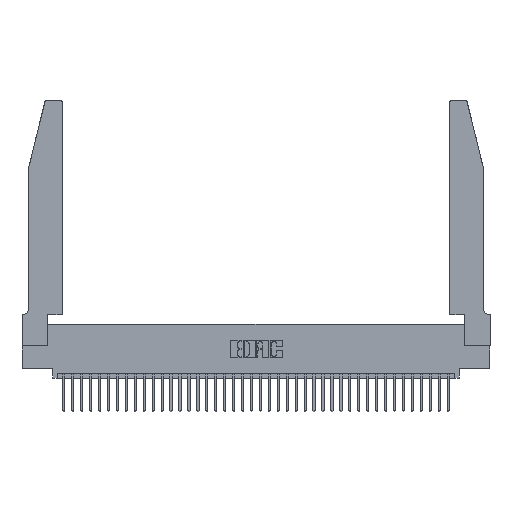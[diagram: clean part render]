
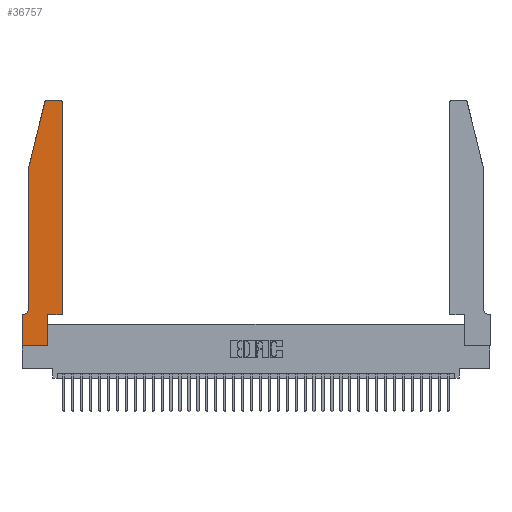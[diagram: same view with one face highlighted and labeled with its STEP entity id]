
A CAD part, top view. The second image highlights one B-rep face of the part: STEP entity #36757.
In plain terms, the highlighted planar face has unit normal (0, 0, 1).
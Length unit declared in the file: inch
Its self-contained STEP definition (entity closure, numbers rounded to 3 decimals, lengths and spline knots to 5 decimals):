
#288 = CARTESIAN_POINT ( 'NONE',  ( 0.0755, 2., 0.37 ) ) ;
#693 = AXIS2_PLACEMENT_3D ( 'NONE', #16150, #37088, #19249 ) ;
#733 = CARTESIAN_POINT ( 'NONE',  ( 0.4505, 0.35, 0.37 ) ) ;
#1399 = LINE ( 'NONE', #6363, #16753 ) ;
#2362 = LINE ( 'NONE', #20560, #8621 ) ;
#2424 = VECTOR ( 'NONE', #24720, 39.37008 ) ;
#2621 = EDGE_CURVE ( 'NONE', #14074, #13895, #5207, .T. ) ;
#3056 = LINE ( 'NONE', #32501, #18376 ) ;
#3131 = VECTOR ( 'NONE', #28277, 39.37008 ) ;
#3741 = VECTOR ( 'NONE', #4279, 39.37008 ) ;
#3900 = CARTESIAN_POINT ( 'NONE',  ( 0.4205, 2.72, 0.37 ) ) ;
#4169 = PLANE ( 'NONE',  #8211 ) ;
#4279 = DIRECTION ( 'NONE',  ( -1., 0., 0. ) ) ;
#4302 = VERTEX_POINT ( 'NONE', #16316 ) ;
#4800 = ORIENTED_EDGE ( 'NONE', *, *, #2621, .T. ) ;
#5201 = CIRCLE ( 'NONE', #34577, 0.03 ) ;
#5207 = LINE ( 'NONE', #32652, #13372 ) ;
#5469 = DIRECTION ( 'NONE',  ( 1., 0., 0. ) ) ;
#5517 = VERTEX_POINT ( 'NONE', #19313 ) ;
#5520 = CARTESIAN_POINT ( 'NONE',  ( 0.4205, 2.75, 0.37 ) ) ;
#5857 = VERTEX_POINT ( 'NONE', #5520 ) ;
#6204 = CARTESIAN_POINT ( 'NONE',  ( 0.0755, 2., 0.37 ) ) ;
#6363 = CARTESIAN_POINT ( 'NONE',  ( 0.4505, 0.35, 0.37 ) ) ;
#6416 = CARTESIAN_POINT ( 'NONE',  ( 0.4505, 0.35, 0.37 ) ) ;
#6497 = EDGE_CURVE ( 'NONE', #18504, #38204, #2362, .T. ) ;
#6819 = ORIENTED_EDGE ( 'NONE', *, *, #9516, .T. ) ;
#6875 = CARTESIAN_POINT ( 'NONE',  ( 0.0055, 0.42, 0.37 ) ) ;
#7000 = DIRECTION ( 'NONE',  ( 1., 0., 0. ) ) ;
#7293 = EDGE_CURVE ( 'NONE', #21320, #4302, #38183, .T. ) ;
#8035 = VECTOR ( 'NONE', #10057, 39.37008 ) ;
#8211 = AXIS2_PLACEMENT_3D ( 'NONE', #25286, #10363, #31402 ) ;
#8336 = ORIENTED_EDGE ( 'NONE', *, *, #17563, .T. ) ;
#8621 = VECTOR ( 'NONE', #5469, 39.37008 ) ;
#9344 = DIRECTION ( 'NONE',  ( 1., 0., 0. ) ) ;
#9454 = ORIENTED_EDGE ( 'NONE', *, *, #32877, .T. ) ;
#9516 = EDGE_CURVE ( 'NONE', #23513, #18504, #33385, .T. ) ;
#9686 = CARTESIAN_POINT ( 'NONE',  ( 0., 0.35, 0.37 ) ) ;
#9973 = DIRECTION ( 'NONE',  ( -1., 0., 0. ) ) ;
#10036 = VECTOR ( 'NONE', #27029, 39.37008 ) ;
#10057 = DIRECTION ( 'NONE',  ( 0., 1., 0. ) ) ;
#10145 = VERTEX_POINT ( 'NONE', #18970 ) ;
#10339 = ORIENTED_EDGE ( 'NONE', *, *, #35412, .T. ) ;
#10363 = DIRECTION ( 'NONE',  ( 0., 0., 1. ) ) ;
#10421 = EDGE_CURVE ( 'NONE', #4302, #23513, #3056, .T. ) ;
#11369 = ORIENTED_EDGE ( 'NONE', *, *, #24259, .T. ) ;
#11918 = LINE ( 'NONE', #31386, #3741 ) ;
#12356 = ORIENTED_EDGE ( 'NONE', *, *, #6497, .T. ) ;
#13372 = VECTOR ( 'NONE', #35670, 39.37008 ) ;
#13895 = VERTEX_POINT ( 'NONE', #6204 ) ;
#14074 = VERTEX_POINT ( 'NONE', #16366 ) ;
#14604 = ORIENTED_EDGE ( 'NONE', *, *, #7293, .T. ) ;
#14616 = VERTEX_POINT ( 'NONE', #6416 ) ;
#15712 = DIRECTION ( 'NONE',  ( -1., 0., 0. ) ) ;
#16150 = CARTESIAN_POINT ( 'NONE',  ( 0.284, 2.72, 0.37 ) ) ;
#16316 = CARTESIAN_POINT ( 'NONE',  ( 0.0055, 0.35, 0.37 ) ) ;
#16366 = CARTESIAN_POINT ( 'NONE',  ( 0.25487, 2.72718, 0.37 ) ) ;
#16753 = VECTOR ( 'NONE', #9344, 39.37008 ) ;
#16895 = ORIENTED_EDGE ( 'NONE', *, *, #10421, .T. ) ;
#16992 = FACE_OUTER_BOUND ( 'NONE', #21462, .T. ) ;
#17351 = AXIS2_PLACEMENT_3D ( 'NONE', #6875, #28031, #9973 ) ;
#17563 = EDGE_CURVE ( 'NONE', #32906, #5857, #5201, .T. ) ;
#18376 = VECTOR ( 'NONE', #15712, 39.37008 ) ;
#18504 = VERTEX_POINT ( 'NONE', #29245 ) ;
#18692 = LINE ( 'NONE', #288, #2424 ) ;
#18970 = CARTESIAN_POINT ( 'NONE',  ( 0.2865, 0.35, 0.37 ) ) ;
#19249 = DIRECTION ( 'NONE',  ( 1., 0., 0. ) ) ;
#19313 = CARTESIAN_POINT ( 'NONE',  ( 0.284, 2.75, 0.37 ) ) ;
#20560 = CARTESIAN_POINT ( 'NONE',  ( 0., 0., 0.37 ) ) ;
#21320 = VERTEX_POINT ( 'NONE', #37100 ) ;
#21462 = EDGE_LOOP ( 'NONE', ( #23441, #11369, #4800, #9454, #14604, #16895, #6819, #12356, #34348, #38389, #10339, #8336 ) ) ;
#21526 = CIRCLE ( 'NONE', #693, 0.03 ) ;
#23441 = ORIENTED_EDGE ( 'NONE', *, *, #38173, .T. ) ;
#23513 = VERTEX_POINT ( 'NONE', #9686 ) ;
#24051 = CARTESIAN_POINT ( 'NONE',  ( 0.2865, 0.35, 0.37 ) ) ;
#24259 = EDGE_CURVE ( 'NONE', #5517, #14074, #21526, .T. ) ;
#24720 = DIRECTION ( 'NONE',  ( 0., -1., 0. ) ) ;
#25150 = DIRECTION ( 'NONE',  ( 0., 0., 1. ) ) ;
#25286 = CARTESIAN_POINT ( 'NONE',  ( 0., 0.35, 0.37 ) ) ;
#25288 = CARTESIAN_POINT ( 'NONE',  ( 0., 0., 0.37 ) ) ;
#27029 = DIRECTION ( 'NONE',  ( 0., 1., 0. ) ) ;
#27841 = CARTESIAN_POINT ( 'NONE',  ( 0.4505, 2.72, 0.37 ) ) ;
#28031 = DIRECTION ( 'NONE',  ( 0., 0., -1. ) ) ;
#28277 = DIRECTION ( 'NONE',  ( 0., -1., 0. ) ) ;
#28765 = CARTESIAN_POINT ( 'NONE',  ( 0.2865, 0., 0.37 ) ) ;
#29245 = CARTESIAN_POINT ( 'NONE',  ( 0., 0., 0.37 ) ) ;
#31386 = CARTESIAN_POINT ( 'NONE',  ( 0.2605, 2.75, 0.37 ) ) ;
#31402 = DIRECTION ( 'NONE',  ( 1., 0., 0. ) ) ;
#32062 = LINE ( 'NONE', #733, #8035 ) ;
#32501 = CARTESIAN_POINT ( 'NONE',  ( 0.0755, 0.35, 0.37 ) ) ;
#32652 = CARTESIAN_POINT ( 'NONE',  ( 0.0755, 2., 0.37 ) ) ;
#32877 = EDGE_CURVE ( 'NONE', #13895, #21320, #18692, .T. ) ;
#32906 = VERTEX_POINT ( 'NONE', #27841 ) ;
#33384 = EDGE_CURVE ( 'NONE', #10145, #14616, #1399, .T. ) ;
#33385 = LINE ( 'NONE', #25288, #3131 ) ;
#33976 = EDGE_CURVE ( 'NONE', #38204, #10145, #33991, .T. ) ;
#33991 = LINE ( 'NONE', #24051, #10036 ) ;
#34348 = ORIENTED_EDGE ( 'NONE', *, *, #33976, .T. ) ;
#34577 = AXIS2_PLACEMENT_3D ( 'NONE', #3900, #25150, #7000 ) ;
#35412 = EDGE_CURVE ( 'NONE', #14616, #32906, #32062, .T. ) ;
#35670 = DIRECTION ( 'NONE',  ( -0.239, -0.971, 0. ) ) ;
#36757 = ADVANCED_FACE ( 'NONE', ( #16992 ), #4169, .T. ) ;
#37088 = DIRECTION ( 'NONE',  ( 0., 0., 1. ) ) ;
#37100 = CARTESIAN_POINT ( 'NONE',  ( 0.0755, 0.42, 0.37 ) ) ;
#38173 = EDGE_CURVE ( 'NONE', #5857, #5517, #11918, .T. ) ;
#38183 = CIRCLE ( 'NONE', #17351, 0.07 ) ;
#38204 = VERTEX_POINT ( 'NONE', #28765 ) ;
#38389 = ORIENTED_EDGE ( 'NONE', *, *, #33384, .T. ) ;
